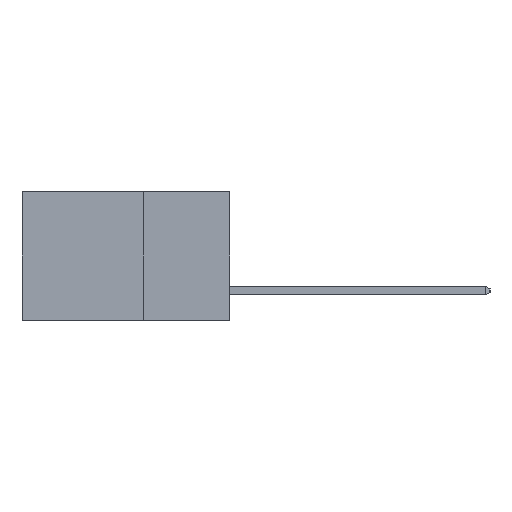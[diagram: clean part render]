
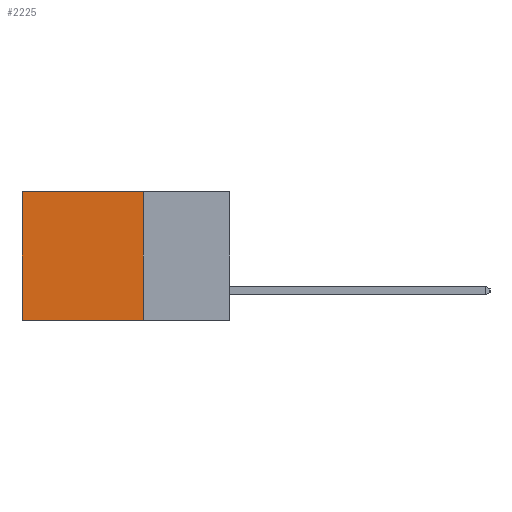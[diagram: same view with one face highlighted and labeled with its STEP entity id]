
A CAD part, left-side view. The second image highlights one B-rep face of the part: STEP entity #2225.
In plain terms, the highlighted planar face has unit normal (-1, 0, 0).
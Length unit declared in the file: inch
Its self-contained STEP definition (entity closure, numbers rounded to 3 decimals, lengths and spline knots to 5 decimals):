
#1637 = DIRECTION ( 'NONE',  ( 1., 0., 0. ) ) ;
#2225 = ADVANCED_FACE ( 'NONE', ( #14325 ), #14649, .F. ) ;
#2924 = CARTESIAN_POINT ( 'NONE',  ( 0.298, 0.25, -0.37 ) ) ;
#3100 = CARTESIAN_POINT ( 'NONE',  ( 0.298, 0.6, 0. ) ) ;
#3305 = VECTOR ( 'NONE', #13997, 39.37008 ) ;
#3660 = VERTEX_POINT ( 'NONE', #17130 ) ;
#3804 = AXIS2_PLACEMENT_3D ( 'NONE', #10115, #1637, #7805 ) ;
#3892 = EDGE_CURVE ( 'NONE', #17378, #6642, #13690, .T. ) ;
#4927 = EDGE_CURVE ( 'NONE', #3660, #17378, #10625, .T. ) ;
#6152 = VECTOR ( 'NONE', #12183, 39.37008 ) ;
#6642 = VERTEX_POINT ( 'NONE', #14718 ) ;
#7805 = DIRECTION ( 'NONE',  ( 0., 0., -1. ) ) ;
#10115 = CARTESIAN_POINT ( 'NONE',  ( 0.298, 0.25, 0. ) ) ;
#10625 = LINE ( 'NONE', #19624, #14384 ) ;
#12046 = LINE ( 'NONE', #12402, #3305 ) ;
#12183 = DIRECTION ( 'NONE',  ( 0., 0., -1. ) ) ;
#12187 = VERTEX_POINT ( 'NONE', #3100 ) ;
#12402 = CARTESIAN_POINT ( 'NONE',  ( 0.298, 0.25, 0. ) ) ;
#13506 = ORIENTED_EDGE ( 'NONE', *, *, #20686, .T. ) ;
#13559 = ORIENTED_EDGE ( 'NONE', *, *, #3892, .F. ) ;
#13690 = LINE ( 'NONE', #15025, #17833 ) ;
#13763 = CARTESIAN_POINT ( 'NONE',  ( 0.298, 0.6, 0. ) ) ;
#13997 = DIRECTION ( 'NONE',  ( 0., 1., 0. ) ) ;
#14325 = FACE_OUTER_BOUND ( 'NONE', #14660, .T. ) ;
#14384 = VECTOR ( 'NONE', #18101, 39.37008 ) ;
#14530 = ORIENTED_EDGE ( 'NONE', *, *, #4927, .F. ) ;
#14649 = PLANE ( 'NONE',  #3804 ) ;
#14660 = EDGE_LOOP ( 'NONE', ( #13506, #13559, #14530, #18925 ) ) ;
#14718 = CARTESIAN_POINT ( 'NONE',  ( 0.298, 0.6, -0.37 ) ) ;
#14849 = EDGE_CURVE ( 'NONE', #3660, #12187, #12046, .T. ) ;
#15025 = CARTESIAN_POINT ( 'NONE',  ( 0.298, 0.25, -0.37 ) ) ;
#17130 = CARTESIAN_POINT ( 'NONE',  ( 0.298, 0.25, 0. ) ) ;
#17378 = VERTEX_POINT ( 'NONE', #2924 ) ;
#17833 = VECTOR ( 'NONE', #18752, 39.37008 ) ;
#18101 = DIRECTION ( 'NONE',  ( 0., 0., -1. ) ) ;
#18752 = DIRECTION ( 'NONE',  ( 0., 1., 0. ) ) ;
#18851 = LINE ( 'NONE', #13763, #6152 ) ;
#18925 = ORIENTED_EDGE ( 'NONE', *, *, #14849, .T. ) ;
#19624 = CARTESIAN_POINT ( 'NONE',  ( 0.298, 0.25, 0. ) ) ;
#20686 = EDGE_CURVE ( 'NONE', #12187, #6642, #18851, .T. ) ;
